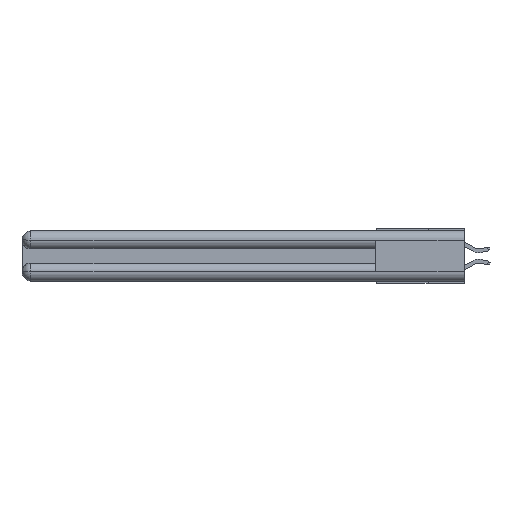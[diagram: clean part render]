
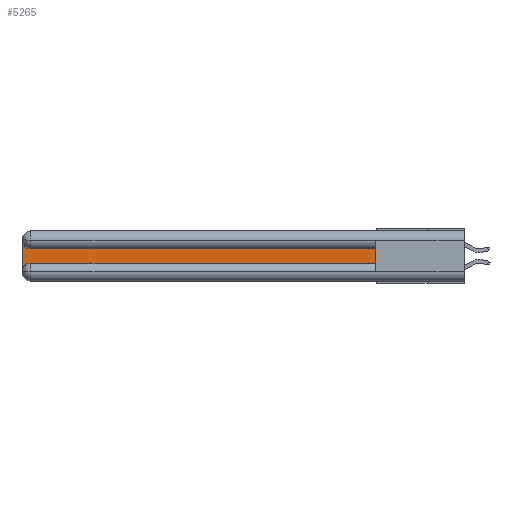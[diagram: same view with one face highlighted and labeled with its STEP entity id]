
A CAD part, left-side view. The second image highlights one B-rep face of the part: STEP entity #5265.
In plain terms, the highlighted planar face has unit normal (-1, 0, 0).
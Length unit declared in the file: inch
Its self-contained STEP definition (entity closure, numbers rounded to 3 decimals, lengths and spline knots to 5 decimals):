
#302 = EDGE_CURVE ( 'NONE', #696, #19157, #27331, .T. ) ;
#482 = VECTOR ( 'NONE', #5940, 39.37008 ) ;
#605 = LINE ( 'NONE', #17288, #21819 ) ;
#696 = VERTEX_POINT ( 'NONE', #6151 ) ;
#754 = EDGE_CURVE ( 'NONE', #15560, #7264, #605, .T. ) ;
#1889 = CARTESIAN_POINT ( 'NONE',  ( 0.075, 2.94, -0.2175 ) ) ;
#2755 = ORIENTED_EDGE ( 'NONE', *, *, #23038, .T. ) ;
#5141 = DIRECTION ( 'NONE',  ( 0., 0., -1. ) ) ;
#5265 = ADVANCED_FACE ( 'NONE', ( #8437 ), #6185, .F. ) ;
#5831 = CARTESIAN_POINT ( 'NONE',  ( 0.075, 3., -0.2175 ) ) ;
#5834 = LINE ( 'NONE', #19913, #13046 ) ;
#5940 = DIRECTION ( 'NONE',  ( 0., -1., 0. ) ) ;
#6151 = CARTESIAN_POINT ( 'NONE',  ( 0.075, 3., -0.2775 ) ) ;
#6185 = PLANE ( 'NONE',  #18324 ) ;
#7264 = VERTEX_POINT ( 'NONE', #11872 ) ;
#7835 = EDGE_CURVE ( 'NONE', #7264, #10911, #5834, .T. ) ;
#8326 = AXIS2_PLACEMENT_3D ( 'NONE', #18563, #27264, #5141 ) ;
#8437 = FACE_OUTER_BOUND ( 'NONE', #17458, .T. ) ;
#8978 = DIRECTION ( 'NONE',  ( 0., 1., 0. ) ) ;
#10066 = LINE ( 'NONE', #16603, #482 ) ;
#10322 = DIRECTION ( 'NONE',  ( 0., 0., -1. ) ) ;
#10911 = VERTEX_POINT ( 'NONE', #27577 ) ;
#11268 = ORIENTED_EDGE ( 'NONE', *, *, #26301, .T. ) ;
#11737 = VECTOR ( 'NONE', #28141, 39.37008 ) ;
#11872 = CARTESIAN_POINT ( 'NONE',  ( 0.075, 0.6, -0.1225 ) ) ;
#12022 = DIRECTION ( 'NONE',  ( 1., 0., 0. ) ) ;
#12844 = CIRCLE ( 'NONE', #27044, 0.06 ) ;
#13046 = VECTOR ( 'NONE', #8978, 39.37008 ) ;
#15014 = CARTESIAN_POINT ( 'NONE',  ( 0.075, 3., -0.1225 ) ) ;
#15560 = VERTEX_POINT ( 'NONE', #28040 ) ;
#16603 = CARTESIAN_POINT ( 'NONE',  ( 0.075, 0.6, -0.2175 ) ) ;
#16873 = LINE ( 'NONE', #5831, #11737 ) ;
#17288 = CARTESIAN_POINT ( 'NONE',  ( 0.075, 0.6, -0.2175 ) ) ;
#17458 = EDGE_LOOP ( 'NONE', ( #21485, #22761, #2755, #22278, #11268, #27326 ) ) ;
#18324 = AXIS2_PLACEMENT_3D ( 'NONE', #15014, #21524, #10322 ) ;
#18563 = CARTESIAN_POINT ( 'NONE',  ( 0.075, 2.94, -0.2775 ) ) ;
#19157 = VERTEX_POINT ( 'NONE', #1889 ) ;
#19913 = CARTESIAN_POINT ( 'NONE',  ( 0.075, 0.6, -0.1225 ) ) ;
#20836 = EDGE_CURVE ( 'NONE', #10911, #21489, #12844, .T. ) ;
#21485 = ORIENTED_EDGE ( 'NONE', *, *, #7835, .T. ) ;
#21489 = VERTEX_POINT ( 'NONE', #24724 ) ;
#21524 = DIRECTION ( 'NONE',  ( 1., 0., 0. ) ) ;
#21819 = VECTOR ( 'NONE', #26183, 39.37008 ) ;
#22278 = ORIENTED_EDGE ( 'NONE', *, *, #302, .T. ) ;
#22761 = ORIENTED_EDGE ( 'NONE', *, *, #20836, .T. ) ;
#23038 = EDGE_CURVE ( 'NONE', #21489, #696, #16873, .T. ) ;
#24724 = CARTESIAN_POINT ( 'NONE',  ( 0.075, 3., -0.0625 ) ) ;
#24973 = DIRECTION ( 'NONE',  ( 0., 0., -1. ) ) ;
#26183 = DIRECTION ( 'NONE',  ( 0., 0., 1. ) ) ;
#26301 = EDGE_CURVE ( 'NONE', #19157, #15560, #10066, .T. ) ;
#26689 = CARTESIAN_POINT ( 'NONE',  ( 0.075, 2.94, -0.0625 ) ) ;
#27044 = AXIS2_PLACEMENT_3D ( 'NONE', #26689, #12022, #24973 ) ;
#27264 = DIRECTION ( 'NONE',  ( 1., 0., 0. ) ) ;
#27326 = ORIENTED_EDGE ( 'NONE', *, *, #754, .T. ) ;
#27331 = CIRCLE ( 'NONE', #8326, 0.06 ) ;
#27577 = CARTESIAN_POINT ( 'NONE',  ( 0.075, 2.94, -0.1225 ) ) ;
#28040 = CARTESIAN_POINT ( 'NONE',  ( 0.075, 0.6, -0.2175 ) ) ;
#28141 = DIRECTION ( 'NONE',  ( 0., 0., -1. ) ) ;
